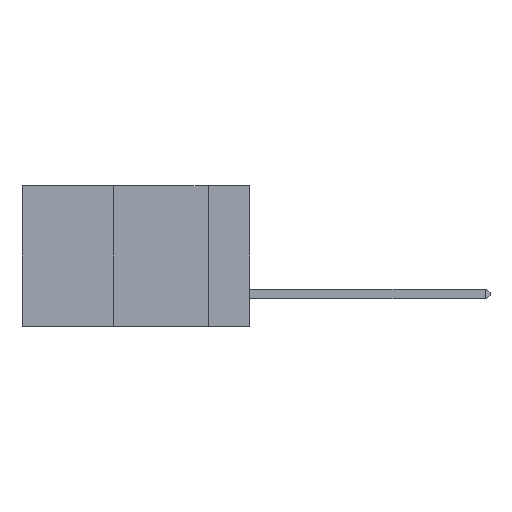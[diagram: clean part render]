
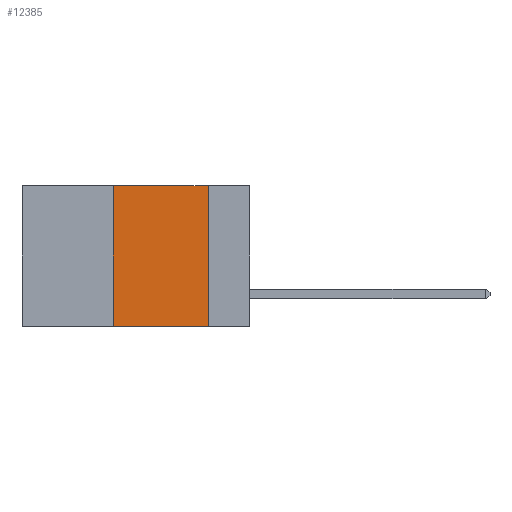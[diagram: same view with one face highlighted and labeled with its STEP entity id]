
A CAD part, left-side view. The second image highlights one B-rep face of the part: STEP entity #12385.
In plain terms, the highlighted planar face has unit normal (-1, 0, 0).
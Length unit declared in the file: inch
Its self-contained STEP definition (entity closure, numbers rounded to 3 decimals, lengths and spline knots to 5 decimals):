
#190 = FACE_OUTER_BOUND ( 'NONE', #14222, .T. ) ;
#987 = EDGE_CURVE ( 'NONE', #9204, #14983, #1983, .T. ) ;
#1485 = CARTESIAN_POINT ( 'NONE',  ( 0., 0.6, 0. ) ) ;
#1983 = LINE ( 'NONE', #1485, #5218 ) ;
#2018 = VECTOR ( 'NONE', #11692, 39.37008 ) ;
#3160 = CARTESIAN_POINT ( 'NONE',  ( 0., 0.11, -0.37 ) ) ;
#4329 = CARTESIAN_POINT ( 'NONE',  ( 0., 0.36, 0. ) ) ;
#4350 = ORIENTED_EDGE ( 'NONE', *, *, #13709, .F. ) ;
#4784 = VERTEX_POINT ( 'NONE', #5880 ) ;
#5218 = VECTOR ( 'NONE', #9719, 39.37008 ) ;
#5606 = LINE ( 'NONE', #14916, #2018 ) ;
#5880 = CARTESIAN_POINT ( 'NONE',  ( 0., 0.36, -0.37 ) ) ;
#6023 = DIRECTION ( 'NONE',  ( 1., 0., 0. ) ) ;
#6494 = DIRECTION ( 'NONE',  ( 0., 0., -1. ) ) ;
#6699 = VERTEX_POINT ( 'NONE', #3160 ) ;
#6775 = AXIS2_PLACEMENT_3D ( 'NONE', #12750, #6023, #13837 ) ;
#6893 = ORIENTED_EDGE ( 'NONE', *, *, #6997, .T. ) ;
#6997 = EDGE_CURVE ( 'NONE', #4784, #6699, #5606, .T. ) ;
#7033 = CARTESIAN_POINT ( 'NONE',  ( 0., 0.11, 0. ) ) ;
#7456 = LINE ( 'NONE', #12375, #10134 ) ;
#7805 = ORIENTED_EDGE ( 'NONE', *, *, #987, .F. ) ;
#9204 = VERTEX_POINT ( 'NONE', #4329 ) ;
#9719 = DIRECTION ( 'NONE',  ( 0., -1., 0. ) ) ;
#10134 = VECTOR ( 'NONE', #13464, 39.37008 ) ;
#10900 = LINE ( 'NONE', #14284, #13804 ) ;
#11512 = EDGE_CURVE ( 'NONE', #4784, #9204, #7456, .T. ) ;
#11692 = DIRECTION ( 'NONE',  ( 0., -1., 0. ) ) ;
#12375 = CARTESIAN_POINT ( 'NONE',  ( 0., 0.36, 0. ) ) ;
#12385 = ADVANCED_FACE ( 'NONE', ( #190 ), #12709, .F. ) ;
#12499 = ORIENTED_EDGE ( 'NONE', *, *, #11512, .F. ) ;
#12709 = PLANE ( 'NONE',  #6775 ) ;
#12750 = CARTESIAN_POINT ( 'NONE',  ( 0., 0.6, 0. ) ) ;
#13464 = DIRECTION ( 'NONE',  ( 0., 0., 1. ) ) ;
#13709 = EDGE_CURVE ( 'NONE', #14983, #6699, #10900, .T. ) ;
#13804 = VECTOR ( 'NONE', #6494, 39.37008 ) ;
#13837 = DIRECTION ( 'NONE',  ( 0., 0., -1. ) ) ;
#14222 = EDGE_LOOP ( 'NONE', ( #4350, #7805, #12499, #6893 ) ) ;
#14284 = CARTESIAN_POINT ( 'NONE',  ( 0., 0.11, 0. ) ) ;
#14916 = CARTESIAN_POINT ( 'NONE',  ( 0., 0.6, -0.37 ) ) ;
#14983 = VERTEX_POINT ( 'NONE', #7033 ) ;
